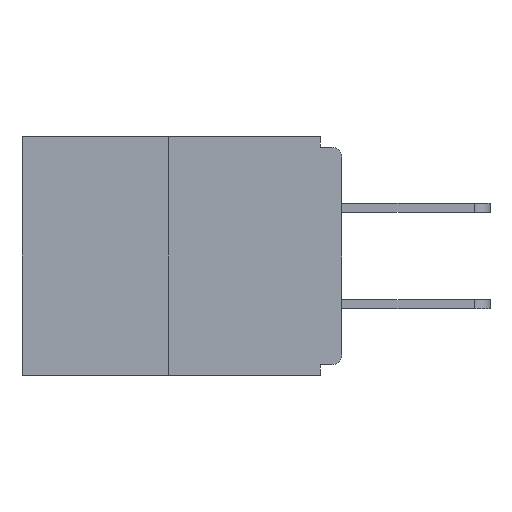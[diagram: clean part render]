
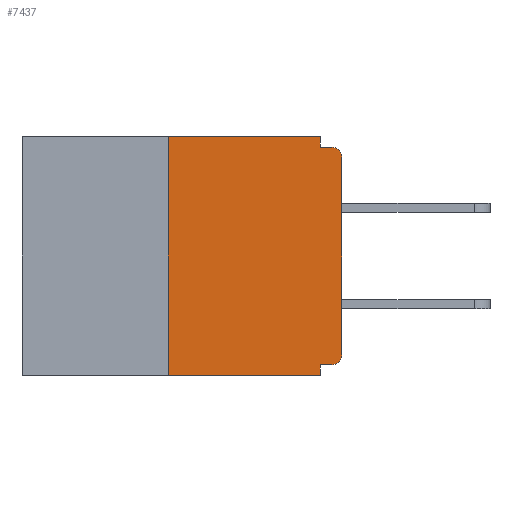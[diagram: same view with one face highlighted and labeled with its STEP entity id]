
A CAD part, left-side view. The second image highlights one B-rep face of the part: STEP entity #7437.
In plain terms, the highlighted planar face has unit normal (-1, 0, 0).
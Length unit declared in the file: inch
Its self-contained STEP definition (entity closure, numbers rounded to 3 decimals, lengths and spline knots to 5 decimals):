
#73 = CARTESIAN_POINT ( 'NONE',  ( 0., 0., -0.03 ) ) ;
#253 = CARTESIAN_POINT ( 'NONE',  ( 0., 0.25, 0. ) ) ;
#799 = VECTOR ( 'NONE', #24372, 39.37008 ) ;
#934 = VERTEX_POINT ( 'NONE', #24696 ) ;
#1517 = EDGE_LOOP ( 'NONE', ( #23376, #13511, #8386, #14620, #18073, #20652, #20606, #1652, #19360, #17028 ) ) ;
#1652 = ORIENTED_EDGE ( 'NONE', *, *, #1772, .T. ) ;
#1772 = EDGE_CURVE ( 'NONE', #27743, #934, #11863, .T. ) ;
#1793 = CARTESIAN_POINT ( 'NONE',  ( 0., 0.031, -0.343 ) ) ;
#2196 = AXIS2_PLACEMENT_3D ( 'NONE', #15487, #20208, #29366 ) ;
#2323 = AXIS2_PLACEMENT_3D ( 'NONE', #6768, #4427, #9073 ) ;
#2370 = CARTESIAN_POINT ( 'NONE',  ( 0., 0.25, 0. ) ) ;
#3242 = AXIS2_PLACEMENT_3D ( 'NONE', #14597, #19123, #21369 ) ;
#3398 = EDGE_CURVE ( 'NONE', #18498, #12710, #16068, .T. ) ;
#4427 = DIRECTION ( 'NONE',  ( -1., 0., 0. ) ) ;
#4672 = VECTOR ( 'NONE', #9413, 39.37008 ) ;
#5059 = CARTESIAN_POINT ( 'NONE',  ( 0., 0., -0.328 ) ) ;
#5225 = EDGE_CURVE ( 'NONE', #16693, #27743, #17728, .T. ) ;
#5759 = VERTEX_POINT ( 'NONE', #7436 ) ;
#6026 = DIRECTION ( 'NONE',  ( 0., 0., -1. ) ) ;
#6611 = DIRECTION ( 'NONE',  ( 0., 0., 1. ) ) ;
#6632 = CARTESIAN_POINT ( 'NONE',  ( 0., 0.46, 0. ) ) ;
#6691 = LINE ( 'NONE', #10022, #14924 ) ;
#6768 = CARTESIAN_POINT ( 'NONE',  ( 0., 0.015, -0.313 ) ) ;
#7436 = CARTESIAN_POINT ( 'NONE',  ( 0., 0.015, -0.328 ) ) ;
#7437 = ADVANCED_FACE ( 'NONE', ( #8911 ), #11286, .F. ) ;
#7644 = DIRECTION ( 'NONE',  ( 0., -1., 0. ) ) ;
#8386 = ORIENTED_EDGE ( 'NONE', *, *, #3398, .T. ) ;
#8911 = FACE_OUTER_BOUND ( 'NONE', #1517, .T. ) ;
#9073 = DIRECTION ( 'NONE',  ( 0., 0., -1. ) ) ;
#9413 = DIRECTION ( 'NONE',  ( 0., 1., 0. ) ) ;
#10022 = CARTESIAN_POINT ( 'NONE',  ( 0., 0., -0.015 ) ) ;
#10688 = LINE ( 'NONE', #5059, #4672 ) ;
#10868 = CARTESIAN_POINT ( 'NONE',  ( 0., 0.031, 0. ) ) ;
#10885 = CARTESIAN_POINT ( 'NONE',  ( 0., 0., 0. ) ) ;
#11286 = PLANE ( 'NONE',  #2196 ) ;
#11863 = CIRCLE ( 'NONE', #3242, 0.015 ) ;
#12039 = CARTESIAN_POINT ( 'NONE',  ( 0., 0.031, -0.328 ) ) ;
#12652 = EDGE_CURVE ( 'NONE', #18498, #16793, #14790, .T. ) ;
#12686 = VECTOR ( 'NONE', #6026, 39.37008 ) ;
#12710 = VERTEX_POINT ( 'NONE', #22923 ) ;
#12714 = CARTESIAN_POINT ( 'NONE',  ( 0., 0.46, -0.343 ) ) ;
#13511 = ORIENTED_EDGE ( 'NONE', *, *, #12652, .F. ) ;
#13601 = EDGE_CURVE ( 'NONE', #5759, #16693, #16478, .T. ) ;
#13682 = CARTESIAN_POINT ( 'NONE',  ( 0., 0., -0.313 ) ) ;
#14154 = LINE ( 'NONE', #10868, #25824 ) ;
#14597 = CARTESIAN_POINT ( 'NONE',  ( 0., 0.015, -0.03 ) ) ;
#14620 = ORIENTED_EDGE ( 'NONE', *, *, #27530, .F. ) ;
#14790 = LINE ( 'NONE', #2370, #22178 ) ;
#14924 = VECTOR ( 'NONE', #7644, 39.37008 ) ;
#15093 = CARTESIAN_POINT ( 'NONE',  ( 0., 0.031, -0.015 ) ) ;
#15487 = CARTESIAN_POINT ( 'NONE',  ( 0., 0.46, 0. ) ) ;
#16068 = LINE ( 'NONE', #12714, #799 ) ;
#16271 = CARTESIAN_POINT ( 'NONE',  ( 0., 0.031, 0. ) ) ;
#16478 = CIRCLE ( 'NONE', #2323, 0.015 ) ;
#16693 = VERTEX_POINT ( 'NONE', #13682 ) ;
#16793 = VERTEX_POINT ( 'NONE', #253 ) ;
#17028 = ORIENTED_EDGE ( 'NONE', *, *, #21001, .F. ) ;
#17728 = LINE ( 'NONE', #10885, #20833 ) ;
#18017 = EDGE_CURVE ( 'NONE', #16793, #21603, #24577, .T. ) ;
#18073 = ORIENTED_EDGE ( 'NONE', *, *, #19649, .F. ) ;
#18498 = VERTEX_POINT ( 'NONE', #29106 ) ;
#19123 = DIRECTION ( 'NONE',  ( -1., 0., 0. ) ) ;
#19360 = ORIENTED_EDGE ( 'NONE', *, *, #26334, .F. ) ;
#19635 = VECTOR ( 'NONE', #20325, 39.37008 ) ;
#19649 = EDGE_CURVE ( 'NONE', #5759, #21521, #10688, .T. ) ;
#19973 = DIRECTION ( 'NONE',  ( 0., 0., -1. ) ) ;
#20208 = DIRECTION ( 'NONE',  ( 1., 0., 0. ) ) ;
#20325 = DIRECTION ( 'NONE',  ( 0., -1., 0. ) ) ;
#20606 = ORIENTED_EDGE ( 'NONE', *, *, #5225, .T. ) ;
#20652 = ORIENTED_EDGE ( 'NONE', *, *, #13601, .T. ) ;
#20833 = VECTOR ( 'NONE', #6611, 39.37008 ) ;
#21001 = EDGE_CURVE ( 'NONE', #21603, #23663, #14154, .T. ) ;
#21369 = DIRECTION ( 'NONE',  ( 0., 0., -1. ) ) ;
#21521 = VERTEX_POINT ( 'NONE', #12039 ) ;
#21603 = VERTEX_POINT ( 'NONE', #16271 ) ;
#22178 = VECTOR ( 'NONE', #22822, 39.37008 ) ;
#22822 = DIRECTION ( 'NONE',  ( 0., 0., 1. ) ) ;
#22923 = CARTESIAN_POINT ( 'NONE',  ( 0., 0.031, -0.343 ) ) ;
#23376 = ORIENTED_EDGE ( 'NONE', *, *, #18017, .F. ) ;
#23663 = VERTEX_POINT ( 'NONE', #15093 ) ;
#24372 = DIRECTION ( 'NONE',  ( 0., -1., 0. ) ) ;
#24577 = LINE ( 'NONE', #6632, #19635 ) ;
#24696 = CARTESIAN_POINT ( 'NONE',  ( 0., 0.015, -0.015 ) ) ;
#25824 = VECTOR ( 'NONE', #19973, 39.37008 ) ;
#26334 = EDGE_CURVE ( 'NONE', #23663, #934, #6691, .T. ) ;
#27530 = EDGE_CURVE ( 'NONE', #21521, #12710, #28307, .T. ) ;
#27743 = VERTEX_POINT ( 'NONE', #73 ) ;
#28307 = LINE ( 'NONE', #1793, #12686 ) ;
#29106 = CARTESIAN_POINT ( 'NONE',  ( 0., 0.25, -0.343 ) ) ;
#29366 = DIRECTION ( 'NONE',  ( 0., 0., -1. ) ) ;
